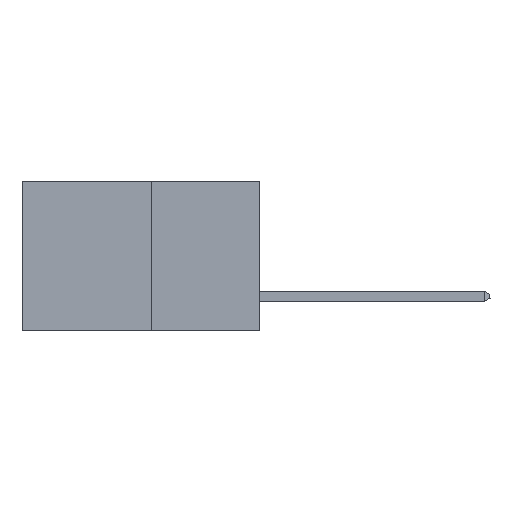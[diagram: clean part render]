
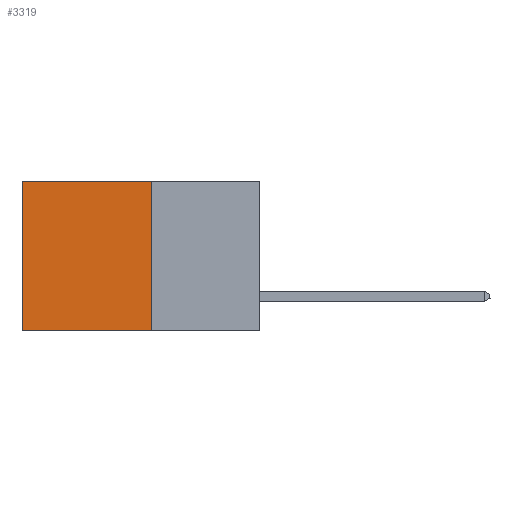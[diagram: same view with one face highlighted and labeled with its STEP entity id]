
A CAD part, left-side view. The second image highlights one B-rep face of the part: STEP entity #3319.
In plain terms, the highlighted planar face has unit normal (-1, 0, 0).
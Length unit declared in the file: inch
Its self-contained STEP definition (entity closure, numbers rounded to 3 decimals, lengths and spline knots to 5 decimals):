
#71 = VECTOR ( 'NONE', #5481, 39.37008 ) ;
#298 = DIRECTION ( 'NONE',  ( 0., 0., -1. ) ) ;
#381 = DIRECTION ( 'NONE',  ( 1., 0., 0. ) ) ;
#1353 = DIRECTION ( 'NONE',  ( 0., 1., 0. ) ) ;
#1611 = VERTEX_POINT ( 'NONE', #10602 ) ;
#2365 = VECTOR ( 'NONE', #15233, 39.37008 ) ;
#2521 = CARTESIAN_POINT ( 'NONE',  ( 0.277, 0.59, -0.37 ) ) ;
#3080 = FACE_OUTER_BOUND ( 'NONE', #8649, .T. ) ;
#3319 = ADVANCED_FACE ( 'NONE', ( #3080 ), #11554, .F. ) ;
#3655 = CARTESIAN_POINT ( 'NONE',  ( 0.277, 0.27, -0.37 ) ) ;
#3681 = VECTOR ( 'NONE', #19349, 39.37008 ) ;
#3785 = CARTESIAN_POINT ( 'NONE',  ( 0.277, 0.27, 0. ) ) ;
#4690 = ORIENTED_EDGE ( 'NONE', *, *, #20780, .F. ) ;
#4863 = LINE ( 'NONE', #3655, #71 ) ;
#5431 = ORIENTED_EDGE ( 'NONE', *, *, #18156, .F. ) ;
#5481 = DIRECTION ( 'NONE',  ( 0., 0., -1. ) ) ;
#6937 = LINE ( 'NONE', #12193, #11196 ) ;
#7592 = VERTEX_POINT ( 'NONE', #3785 ) ;
#8074 = ORIENTED_EDGE ( 'NONE', *, *, #17488, .T. ) ;
#8649 = EDGE_LOOP ( 'NONE', ( #11354, #5431, #4690, #8074 ) ) ;
#9773 = CARTESIAN_POINT ( 'NONE',  ( 0.277, 0.27, -0.37 ) ) ;
#10602 = CARTESIAN_POINT ( 'NONE',  ( 0.277, 0.59, -0.37 ) ) ;
#10880 = LINE ( 'NONE', #2521, #2365 ) ;
#11196 = VECTOR ( 'NONE', #1353, 39.37008 ) ;
#11354 = ORIENTED_EDGE ( 'NONE', *, *, #15217, .T. ) ;
#11554 = PLANE ( 'NONE',  #12046 ) ;
#12046 = AXIS2_PLACEMENT_3D ( 'NONE', #9773, #381, #298 ) ;
#12193 = CARTESIAN_POINT ( 'NONE',  ( 0.277, 0.27, -0.37 ) ) ;
#13180 = VERTEX_POINT ( 'NONE', #18743 ) ;
#13364 = LINE ( 'NONE', #17551, #3681 ) ;
#15217 = EDGE_CURVE ( 'NONE', #20728, #1611, #10880, .T. ) ;
#15233 = DIRECTION ( 'NONE',  ( 0., 0., -1. ) ) ;
#15403 = CARTESIAN_POINT ( 'NONE',  ( 0.277, 0.59, 0. ) ) ;
#17488 = EDGE_CURVE ( 'NONE', #7592, #20728, #13364, .T. ) ;
#17551 = CARTESIAN_POINT ( 'NONE',  ( 0.277, 0.27, 0. ) ) ;
#18156 = EDGE_CURVE ( 'NONE', #13180, #1611, #6937, .T. ) ;
#18743 = CARTESIAN_POINT ( 'NONE',  ( 0.277, 0.27, -0.37 ) ) ;
#19349 = DIRECTION ( 'NONE',  ( 0., 1., 0. ) ) ;
#20728 = VERTEX_POINT ( 'NONE', #15403 ) ;
#20780 = EDGE_CURVE ( 'NONE', #7592, #13180, #4863, .T. ) ;
